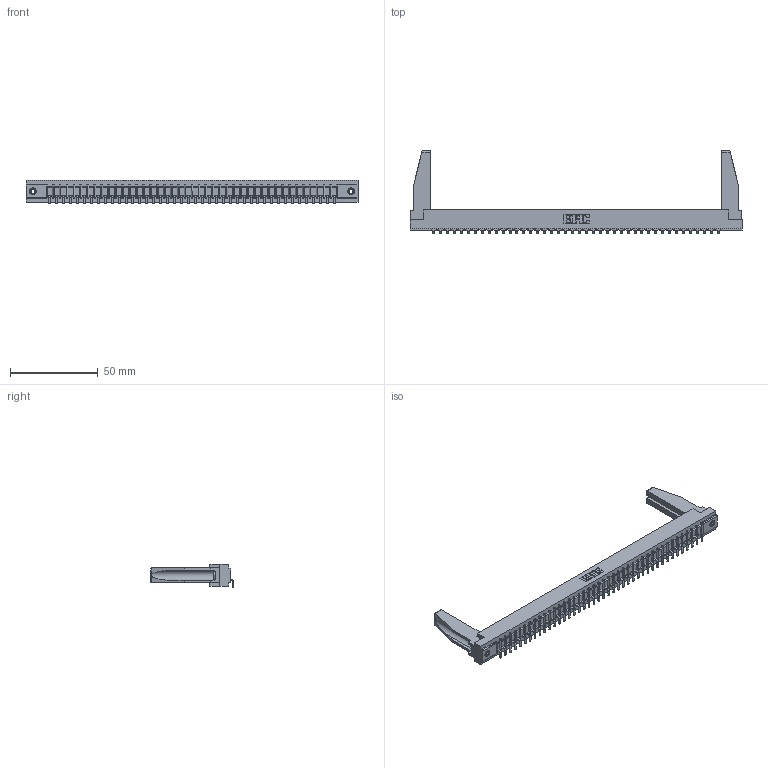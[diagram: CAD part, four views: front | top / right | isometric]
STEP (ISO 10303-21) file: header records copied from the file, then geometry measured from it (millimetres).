
FILE_DESCRIPTION (( 'STEP AP203' ), '1' );
FILE_NAME ('357-042-553-178.STEP', '2019-09-17T10:31:37', ( '' ), ( '' ), 'SwSTEP 2.0', 'SolidWorks 2016', '' );
FILE_SCHEMA (( 'CONFIG_CONTROL_DESIGN' ));
Length unit declared in the file: inch
Products named in the file (5): 307-290-002_553; 345-250-001_345-250-001-102; 307-220-078; 307 Part_.156 Dia Mounting Holes; 357-042-553-178
Assembly tree (47 placements, depth 2):
  357-042-553-178
    307 Part_.156 Dia Mounting Holes
    307-290-002_553  x42
    307-220-078  x2
    345-250-001_345-250-001-102  x2
Bounding box: 189.43 x 47.03 x 13.5 mm (x, y, z)
Volume: 24264.9 mm3; surface area: 29306.9 mm2
Topology: 47 solids, 47 shells, 3567 faces, 10901 edges, 7142 vertices
Faces by surface type: plane 2128, cylinder 1337, sphere 86, cone 12, torus 4
Entity records: 39299 total; most frequent: CARTESIAN_POINT 6630, ORIENTED_EDGE 6576, DIRECTION 6398, EDGE_CURVE 3288, LINE 2522, VECTOR 2522, VERTEX_POINT 2128, AXIS2_PLACEMENT_3D 1938
